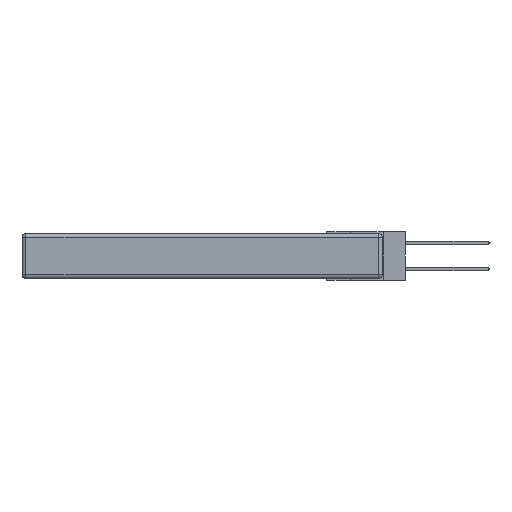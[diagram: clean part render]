
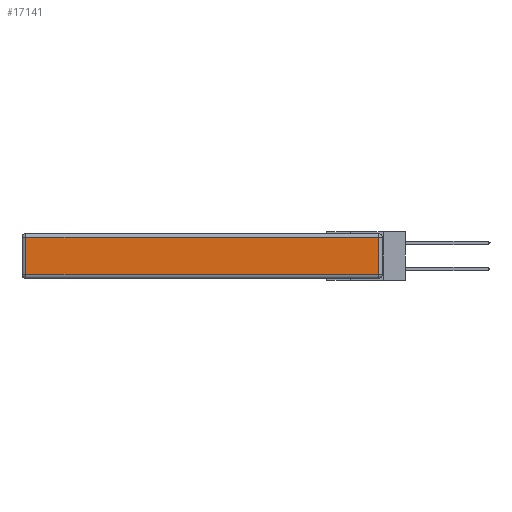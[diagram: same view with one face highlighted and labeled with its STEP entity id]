
A CAD part, left-side view. The second image highlights one B-rep face of the part: STEP entity #17141.
In plain terms, the highlighted planar face has unit normal (-1, 0, 0).
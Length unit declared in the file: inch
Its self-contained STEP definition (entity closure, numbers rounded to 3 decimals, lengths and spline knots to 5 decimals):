
#563 = VERTEX_POINT ( 'NONE', #2995 ) ;
#743 = EDGE_CURVE ( 'NONE', #15821, #2878, #6959, .T. ) ;
#913 = VECTOR ( 'NONE', #7549, 39.37008 ) ;
#1964 = DIRECTION ( 'NONE',  ( 0., -1., 0. ) ) ;
#2554 = AXIS2_PLACEMENT_3D ( 'NONE', #11912, #11973, #13285 ) ;
#2618 = VECTOR ( 'NONE', #16978, 39.37008 ) ;
#2878 = VERTEX_POINT ( 'NONE', #15239 ) ;
#2995 = CARTESIAN_POINT ( 'NONE',  ( 0., 2.72, -0.03 ) ) ;
#4008 = ORIENTED_EDGE ( 'NONE', *, *, #14631, .T. ) ;
#4888 = VERTEX_POINT ( 'NONE', #8161 ) ;
#6959 = LINE ( 'NONE', #10774, #15989 ) ;
#7040 = EDGE_CURVE ( 'NONE', #4888, #15821, #16284, .T. ) ;
#7549 = DIRECTION ( 'NONE',  ( 0., 1., 0. ) ) ;
#8080 = EDGE_CURVE ( 'NONE', #2878, #563, #16877, .T. ) ;
#8161 = CARTESIAN_POINT ( 'NONE',  ( 0., 2.72, -0.313 ) ) ;
#8194 = ORIENTED_EDGE ( 'NONE', *, *, #7040, .T. ) ;
#10245 = CARTESIAN_POINT ( 'NONE',  ( 0., 2.72, -0.343 ) ) ;
#10540 = DIRECTION ( 'NONE',  ( 0., 0., 1. ) ) ;
#10617 = PLANE ( 'NONE',  #2554 ) ;
#10774 = CARTESIAN_POINT ( 'NONE',  ( 0., 0.03, -0.343 ) ) ;
#11638 = CARTESIAN_POINT ( 'NONE',  ( 0., 2.75, -0.03 ) ) ;
#11912 = CARTESIAN_POINT ( 'NONE',  ( 0., 0., -0.343 ) ) ;
#11973 = DIRECTION ( 'NONE',  ( -1., 0., 0. ) ) ;
#13285 = DIRECTION ( 'NONE',  ( 0., 0., 1. ) ) ;
#13515 = ORIENTED_EDGE ( 'NONE', *, *, #8080, .T. ) ;
#14039 = CARTESIAN_POINT ( 'NONE',  ( 0., 0., -0.313 ) ) ;
#14083 = EDGE_LOOP ( 'NONE', ( #8194, #15776, #13515, #4008 ) ) ;
#14420 = LINE ( 'NONE', #10245, #2618 ) ;
#14631 = EDGE_CURVE ( 'NONE', #563, #4888, #14420, .T. ) ;
#15239 = CARTESIAN_POINT ( 'NONE',  ( 0., 0.03, -0.03 ) ) ;
#15547 = CARTESIAN_POINT ( 'NONE',  ( 0., 0.03, -0.313 ) ) ;
#15776 = ORIENTED_EDGE ( 'NONE', *, *, #743, .T. ) ;
#15821 = VERTEX_POINT ( 'NONE', #15547 ) ;
#15989 = VECTOR ( 'NONE', #10540, 39.37008 ) ;
#15993 = FACE_OUTER_BOUND ( 'NONE', #14083, .T. ) ;
#16284 = LINE ( 'NONE', #14039, #16495 ) ;
#16495 = VECTOR ( 'NONE', #1964, 39.37008 ) ;
#16877 = LINE ( 'NONE', #11638, #913 ) ;
#16978 = DIRECTION ( 'NONE',  ( 0., 0., -1. ) ) ;
#17141 = ADVANCED_FACE ( 'NONE', ( #15993 ), #10617, .T. ) ;
